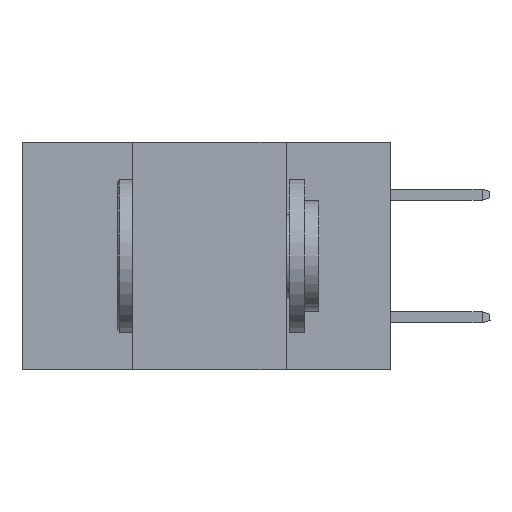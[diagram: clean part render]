
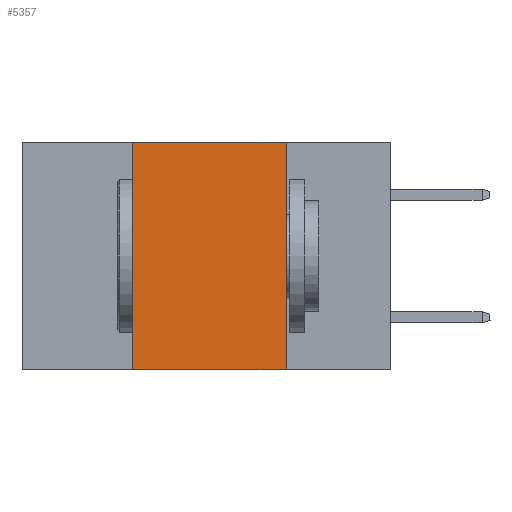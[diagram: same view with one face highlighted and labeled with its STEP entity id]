
A CAD part, left-side view. The second image highlights one B-rep face of the part: STEP entity #5357.
In plain terms, the highlighted planar face has unit normal (-1, 0, 0).
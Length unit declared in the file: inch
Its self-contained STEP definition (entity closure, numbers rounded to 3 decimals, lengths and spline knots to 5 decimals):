
#559 = CARTESIAN_POINT ( 'NONE',  ( 0., 0.42, 0. ) ) ;
#639 = VECTOR ( 'NONE', #3231, 39.37008 ) ;
#641 = PLANE ( 'NONE',  #9732 ) ;
#1076 = VECTOR ( 'NONE', #4123, 39.37008 ) ;
#1565 = ORIENTED_EDGE ( 'NONE', *, *, #6757, .T. ) ;
#1845 = VERTEX_POINT ( 'NONE', #7655 ) ;
#3231 = DIRECTION ( 'NONE',  ( 0., -1., 0. ) ) ;
#3378 = DIRECTION ( 'NONE',  ( 0., 0., -1. ) ) ;
#3572 = VERTEX_POINT ( 'NONE', #7041 ) ;
#4123 = DIRECTION ( 'NONE',  ( 0., -1., 0. ) ) ;
#4291 = VERTEX_POINT ( 'NONE', #11057 ) ;
#4451 = VECTOR ( 'NONE', #12508, 39.37008 ) ;
#5357 = ADVANCED_FACE ( 'NONE', ( #7822 ), #641, .F. ) ;
#6004 = ORIENTED_EDGE ( 'NONE', *, *, #12781, .F. ) ;
#6667 = ORIENTED_EDGE ( 'NONE', *, *, #6885, .F. ) ;
#6757 = EDGE_CURVE ( 'NONE', #1845, #4291, #11330, .T. ) ;
#6885 = EDGE_CURVE ( 'NONE', #1845, #7695, #9120, .T. ) ;
#7041 = CARTESIAN_POINT ( 'NONE',  ( 0., 0.17, 0. ) ) ;
#7358 = LINE ( 'NONE', #7392, #7515 ) ;
#7392 = CARTESIAN_POINT ( 'NONE',  ( 0., 0.17, 0. ) ) ;
#7439 = EDGE_LOOP ( 'NONE', ( #8437, #6004, #6667, #1565 ) ) ;
#7515 = VECTOR ( 'NONE', #3378, 39.37008 ) ;
#7540 = LINE ( 'NONE', #11836, #1076 ) ;
#7655 = CARTESIAN_POINT ( 'NONE',  ( 0., 0.42, -0.37 ) ) ;
#7695 = VERTEX_POINT ( 'NONE', #559 ) ;
#7822 = FACE_OUTER_BOUND ( 'NONE', #7439, .T. ) ;
#8437 = ORIENTED_EDGE ( 'NONE', *, *, #8785, .F. ) ;
#8717 = CARTESIAN_POINT ( 'NONE',  ( 0., 0.6, 0. ) ) ;
#8785 = EDGE_CURVE ( 'NONE', #3572, #4291, #7358, .T. ) ;
#9120 = LINE ( 'NONE', #11359, #4451 ) ;
#9716 = DIRECTION ( 'NONE',  ( 1., 0., 0. ) ) ;
#9732 = AXIS2_PLACEMENT_3D ( 'NONE', #8717, #9716, #11634 ) ;
#10276 = CARTESIAN_POINT ( 'NONE',  ( 0., 0.6, -0.37 ) ) ;
#11057 = CARTESIAN_POINT ( 'NONE',  ( 0., 0.17, -0.37 ) ) ;
#11330 = LINE ( 'NONE', #10276, #639 ) ;
#11359 = CARTESIAN_POINT ( 'NONE',  ( 0., 0.42, 0. ) ) ;
#11634 = DIRECTION ( 'NONE',  ( 0., 0., -1. ) ) ;
#11836 = CARTESIAN_POINT ( 'NONE',  ( 0., 0.6, 0. ) ) ;
#12508 = DIRECTION ( 'NONE',  ( 0., 0., 1. ) ) ;
#12781 = EDGE_CURVE ( 'NONE', #7695, #3572, #7540, .T. ) ;
